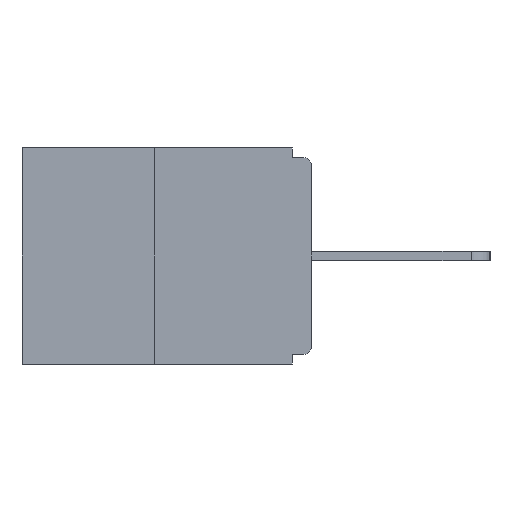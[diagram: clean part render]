
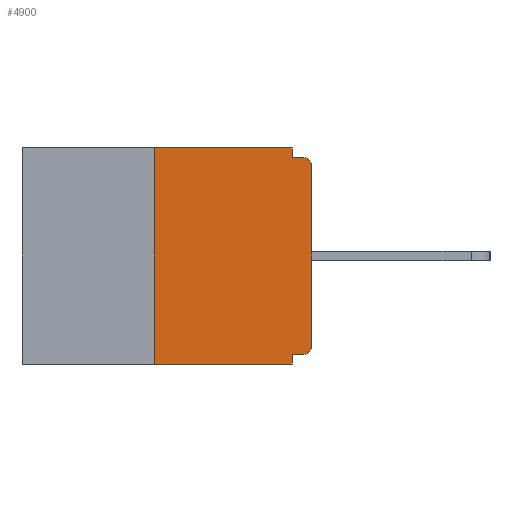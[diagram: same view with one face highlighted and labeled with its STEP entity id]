
A CAD part, left-side view. The second image highlights one B-rep face of the part: STEP entity #4900.
In plain terms, the highlighted planar face has unit normal (-1, 0, 0).
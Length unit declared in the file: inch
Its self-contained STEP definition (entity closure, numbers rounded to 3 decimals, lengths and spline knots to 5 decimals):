
#21 = DIRECTION ( 'NONE',  ( 0., 0., -1. ) ) ;
#311 = ORIENTED_EDGE ( 'NONE', *, *, #1017, .F. ) ;
#347 = EDGE_CURVE ( 'NONE', #22774, #10390, #13607, .T. ) ;
#425 = EDGE_CURVE ( 'NONE', #16407, #13985, #17418, .T. ) ;
#469 = CARTESIAN_POINT ( 'NONE',  ( 0., 0.25, -0.343 ) ) ;
#1017 = EDGE_CURVE ( 'NONE', #24607, #2822, #10618, .T. ) ;
#1096 = ORIENTED_EDGE ( 'NONE', *, *, #23981, .F. ) ;
#1607 = VECTOR ( 'NONE', #10749, 39.37008 ) ;
#1972 = ORIENTED_EDGE ( 'NONE', *, *, #8494, .T. ) ;
#1980 = CIRCLE ( 'NONE', #19576, 0.015 ) ;
#2027 = CARTESIAN_POINT ( 'NONE',  ( 0., 0.031, -0.015 ) ) ;
#2162 = ORIENTED_EDGE ( 'NONE', *, *, #347, .F. ) ;
#2278 = DIRECTION ( 'NONE',  ( 0., 0., -1. ) ) ;
#2463 = CARTESIAN_POINT ( 'NONE',  ( 0., 0.015, -0.328 ) ) ;
#2677 = VECTOR ( 'NONE', #21, 39.37008 ) ;
#2822 = VERTEX_POINT ( 'NONE', #2027 ) ;
#3229 = ORIENTED_EDGE ( 'NONE', *, *, #12080, .T. ) ;
#3645 = VERTEX_POINT ( 'NONE', #20452 ) ;
#3711 = DIRECTION ( 'NONE',  ( -1., 0., 0. ) ) ;
#4286 = LINE ( 'NONE', #20031, #14635 ) ;
#4610 = CARTESIAN_POINT ( 'NONE',  ( 0., 0.25, 0. ) ) ;
#4674 = DIRECTION ( 'NONE',  ( 0., 1., 0. ) ) ;
#4870 = ORIENTED_EDGE ( 'NONE', *, *, #12923, .F. ) ;
#4900 = ADVANCED_FACE ( 'NONE', ( #17680 ), #7973, .F. ) ;
#5231 = LINE ( 'NONE', #8958, #1607 ) ;
#6298 = CARTESIAN_POINT ( 'NONE',  ( 0., 0., -0.03 ) ) ;
#6345 = EDGE_CURVE ( 'NONE', #13985, #7002, #7642, .T. ) ;
#6401 = DIRECTION ( 'NONE',  ( 0., 0., 1. ) ) ;
#7002 = VERTEX_POINT ( 'NONE', #20041 ) ;
#7076 = CARTESIAN_POINT ( 'NONE',  ( 0., 0.46, 0. ) ) ;
#7642 = CIRCLE ( 'NONE', #12561, 0.015 ) ;
#7866 = EDGE_CURVE ( 'NONE', #21980, #22774, #4286, .T. ) ;
#7973 = PLANE ( 'NONE',  #13588 ) ;
#8494 = EDGE_CURVE ( 'NONE', #21980, #16407, #1980, .T. ) ;
#8741 = DIRECTION ( 'NONE',  ( 0., -1., 0. ) ) ;
#8958 = CARTESIAN_POINT ( 'NONE',  ( 0., 0.46, -0.343 ) ) ;
#9107 = VERTEX_POINT ( 'NONE', #469 ) ;
#9230 = LINE ( 'NONE', #7076, #12878 ) ;
#10140 = DIRECTION ( 'NONE',  ( 0., 0., 1. ) ) ;
#10390 = VERTEX_POINT ( 'NONE', #12191 ) ;
#10571 = ORIENTED_EDGE ( 'NONE', *, *, #7866, .F. ) ;
#10618 = LINE ( 'NONE', #16484, #13990 ) ;
#10749 = DIRECTION ( 'NONE',  ( 0., -1., 0. ) ) ;
#11993 = EDGE_CURVE ( 'NONE', #9107, #3645, #21751, .T. ) ;
#12068 = DIRECTION ( 'NONE',  ( 0., 0., -1. ) ) ;
#12080 = EDGE_CURVE ( 'NONE', #9107, #10390, #5231, .T. ) ;
#12111 = CARTESIAN_POINT ( 'NONE',  ( 0., 0.031, -0.328 ) ) ;
#12191 = CARTESIAN_POINT ( 'NONE',  ( 0., 0.031, -0.343 ) ) ;
#12561 = AXIS2_PLACEMENT_3D ( 'NONE', #22786, #18455, #18958 ) ;
#12878 = VECTOR ( 'NONE', #8741, 39.37008 ) ;
#12923 = EDGE_CURVE ( 'NONE', #2822, #7002, #24358, .T. ) ;
#13334 = ORIENTED_EDGE ( 'NONE', *, *, #425, .T. ) ;
#13588 = AXIS2_PLACEMENT_3D ( 'NONE', #17931, #15755, #12068 ) ;
#13607 = LINE ( 'NONE', #25223, #2677 ) ;
#13720 = CARTESIAN_POINT ( 'NONE',  ( 0., 0., 0. ) ) ;
#13985 = VERTEX_POINT ( 'NONE', #6298 ) ;
#13990 = VECTOR ( 'NONE', #24293, 39.37008 ) ;
#14635 = VECTOR ( 'NONE', #4674, 39.37008 ) ;
#15316 = CARTESIAN_POINT ( 'NONE',  ( 0., 0.031, 0. ) ) ;
#15674 = ORIENTED_EDGE ( 'NONE', *, *, #6345, .T. ) ;
#15755 = DIRECTION ( 'NONE',  ( 1., 0., 0. ) ) ;
#16407 = VERTEX_POINT ( 'NONE', #23657 ) ;
#16484 = CARTESIAN_POINT ( 'NONE',  ( 0., 0.031, 0. ) ) ;
#17166 = ORIENTED_EDGE ( 'NONE', *, *, #11993, .F. ) ;
#17418 = LINE ( 'NONE', #13720, #19034 ) ;
#17680 = FACE_OUTER_BOUND ( 'NONE', #21225, .T. ) ;
#17931 = CARTESIAN_POINT ( 'NONE',  ( 0., 0.46, 0. ) ) ;
#18342 = CARTESIAN_POINT ( 'NONE',  ( 0., 0., -0.015 ) ) ;
#18455 = DIRECTION ( 'NONE',  ( -1., 0., 0. ) ) ;
#18958 = DIRECTION ( 'NONE',  ( 0., 0., -1. ) ) ;
#19034 = VECTOR ( 'NONE', #10140, 39.37008 ) ;
#19210 = VECTOR ( 'NONE', #22440, 39.37008 ) ;
#19574 = VECTOR ( 'NONE', #6401, 39.37008 ) ;
#19576 = AXIS2_PLACEMENT_3D ( 'NONE', #21472, #3711, #2278 ) ;
#20031 = CARTESIAN_POINT ( 'NONE',  ( 0., 0., -0.328 ) ) ;
#20041 = CARTESIAN_POINT ( 'NONE',  ( 0., 0.015, -0.015 ) ) ;
#20452 = CARTESIAN_POINT ( 'NONE',  ( 0., 0.25, 0. ) ) ;
#21225 = EDGE_LOOP ( 'NONE', ( #1096, #17166, #3229, #2162, #10571, #1972, #13334, #15674, #4870, #311 ) ) ;
#21472 = CARTESIAN_POINT ( 'NONE',  ( 0., 0.015, -0.313 ) ) ;
#21751 = LINE ( 'NONE', #4610, #19574 ) ;
#21980 = VERTEX_POINT ( 'NONE', #2463 ) ;
#22440 = DIRECTION ( 'NONE',  ( 0., -1., 0. ) ) ;
#22774 = VERTEX_POINT ( 'NONE', #12111 ) ;
#22786 = CARTESIAN_POINT ( 'NONE',  ( 0., 0.015, -0.03 ) ) ;
#23657 = CARTESIAN_POINT ( 'NONE',  ( 0., 0., -0.313 ) ) ;
#23981 = EDGE_CURVE ( 'NONE', #3645, #24607, #9230, .T. ) ;
#24293 = DIRECTION ( 'NONE',  ( 0., 0., -1. ) ) ;
#24358 = LINE ( 'NONE', #18342, #19210 ) ;
#24607 = VERTEX_POINT ( 'NONE', #15316 ) ;
#25223 = CARTESIAN_POINT ( 'NONE',  ( 0., 0.031, -0.343 ) ) ;
